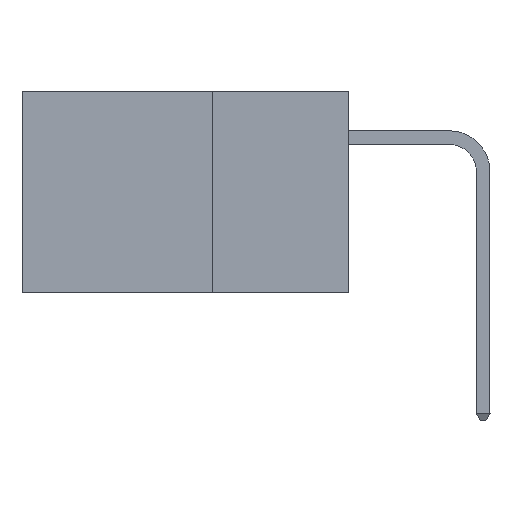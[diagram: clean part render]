
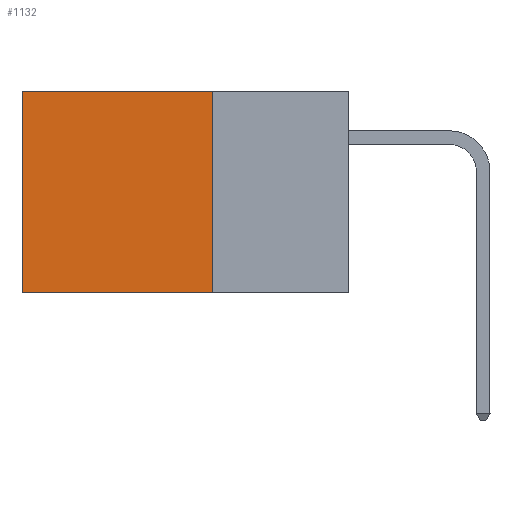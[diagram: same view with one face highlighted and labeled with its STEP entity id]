
A CAD part, left-side view. The second image highlights one B-rep face of the part: STEP entity #1132.
In plain terms, the highlighted planar face has unit normal (-1, 0, 0).
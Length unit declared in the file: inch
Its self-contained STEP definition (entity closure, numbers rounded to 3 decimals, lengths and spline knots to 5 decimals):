
#936 = AXIS2_PLACEMENT_3D ( 'NONE', #5287, #9098, #11448 ) ;
#1132 = ADVANCED_FACE ( 'NONE', ( #6510 ), #14210, .F. ) ;
#1194 = VERTEX_POINT ( 'NONE', #10395 ) ;
#1207 = EDGE_CURVE ( 'NONE', #1194, #8281, #3079, .T. ) ;
#2028 = CARTESIAN_POINT ( 'NONE',  ( 0.2875, 0.25, -0.37 ) ) ;
#2249 = EDGE_CURVE ( 'NONE', #12099, #9256, #6204, .T. ) ;
#3079 = LINE ( 'NONE', #4070, #7460 ) ;
#3222 = LINE ( 'NONE', #5578, #10725 ) ;
#3417 = ORIENTED_EDGE ( 'NONE', *, *, #2249, .T. ) ;
#4070 = CARTESIAN_POINT ( 'NONE',  ( 0.2875, 0.25, 0. ) ) ;
#4482 = CARTESIAN_POINT ( 'NONE',  ( 0.2875, 0.6, 0. ) ) ;
#5287 = CARTESIAN_POINT ( 'NONE',  ( 0.2875, 0.25, 0. ) ) ;
#5366 = DIRECTION ( 'NONE',  ( 0., 0., -1. ) ) ;
#5578 = CARTESIAN_POINT ( 'NONE',  ( 0.2875, 0.25, 0. ) ) ;
#5786 = ORIENTED_EDGE ( 'NONE', *, *, #1207, .F. ) ;
#6204 = LINE ( 'NONE', #11074, #13249 ) ;
#6510 = FACE_OUTER_BOUND ( 'NONE', #13967, .T. ) ;
#7460 = VECTOR ( 'NONE', #5366, 39.37008 ) ;
#7877 = ORIENTED_EDGE ( 'NONE', *, *, #12889, .T. ) ;
#8012 = DIRECTION ( 'NONE',  ( 0., 1., 0. ) ) ;
#8281 = VERTEX_POINT ( 'NONE', #2028 ) ;
#9098 = DIRECTION ( 'NONE',  ( 1., 0., 0. ) ) ;
#9256 = VERTEX_POINT ( 'NONE', #13192 ) ;
#10395 = CARTESIAN_POINT ( 'NONE',  ( 0.2875, 0.25, 0. ) ) ;
#10725 = VECTOR ( 'NONE', #8012, 39.37008 ) ;
#10790 = DIRECTION ( 'NONE',  ( 0., 1., 0. ) ) ;
#11074 = CARTESIAN_POINT ( 'NONE',  ( 0.2875, 0.6, 0. ) ) ;
#11448 = DIRECTION ( 'NONE',  ( 0., 0., -1. ) ) ;
#11910 = CARTESIAN_POINT ( 'NONE',  ( 0.2875, 0.25, -0.37 ) ) ;
#12031 = VECTOR ( 'NONE', #10790, 39.37008 ) ;
#12099 = VERTEX_POINT ( 'NONE', #4482 ) ;
#12436 = DIRECTION ( 'NONE',  ( 0., 0., -1. ) ) ;
#12889 = EDGE_CURVE ( 'NONE', #1194, #12099, #3222, .T. ) ;
#13192 = CARTESIAN_POINT ( 'NONE',  ( 0.2875, 0.6, -0.37 ) ) ;
#13249 = VECTOR ( 'NONE', #12436, 39.37008 ) ;
#13875 = ORIENTED_EDGE ( 'NONE', *, *, #15939, .F. ) ;
#13967 = EDGE_LOOP ( 'NONE', ( #3417, #13875, #5786, #7877 ) ) ;
#14210 = PLANE ( 'NONE',  #936 ) ;
#14754 = LINE ( 'NONE', #11910, #12031 ) ;
#15939 = EDGE_CURVE ( 'NONE', #8281, #9256, #14754, .T. ) ;
